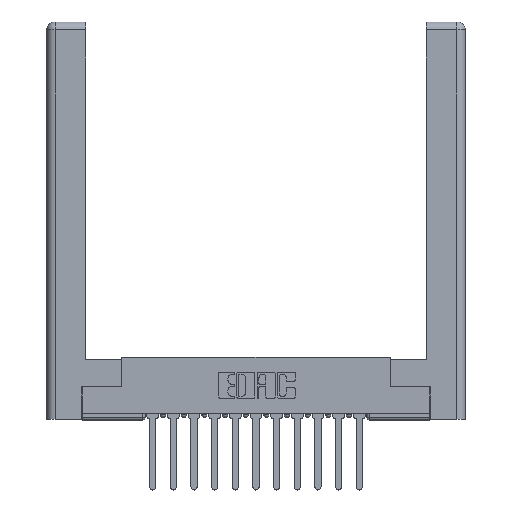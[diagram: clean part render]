
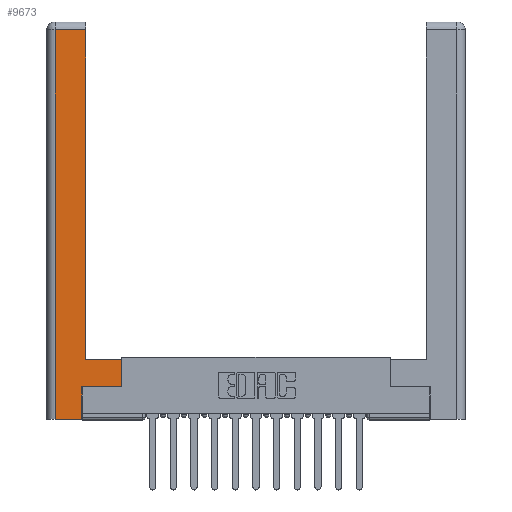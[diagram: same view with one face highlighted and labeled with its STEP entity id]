
A CAD part, top view. The second image highlights one B-rep face of the part: STEP entity #9673.
In plain terms, the highlighted planar face has unit normal (0, 0, 1).
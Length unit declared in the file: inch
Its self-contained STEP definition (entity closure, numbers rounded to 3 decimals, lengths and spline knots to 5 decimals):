
#400 = CARTESIAN_POINT ( 'NONE',  ( 0.565, 0.245, 0. ) ) ;
#1052 = DIRECTION ( 'NONE',  ( 0., 1., 0. ) ) ;
#1970 = CARTESIAN_POINT ( 'NONE',  ( 0.265, 0., 0. ) ) ;
#2134 = DIRECTION ( 'NONE',  ( 0., 1., 0. ) ) ;
#2205 = ORIENTED_EDGE ( 'NONE', *, *, #2290, .T. ) ;
#2249 = EDGE_CURVE ( 'NONE', #7767, #11733, #14508, .T. ) ;
#2290 = EDGE_CURVE ( 'NONE', #13692, #11675, #14270, .T. ) ;
#2493 = CARTESIAN_POINT ( 'NONE',  ( 0.565, 0.45, 0. ) ) ;
#2501 = CARTESIAN_POINT ( 'NONE',  ( 0.0615, 0., 0. ) ) ;
#3147 = EDGE_CURVE ( 'NONE', #8965, #13692, #14709, .T. ) ;
#3248 = FACE_OUTER_BOUND ( 'NONE', #9506, .T. ) ;
#3335 = DIRECTION ( 'NONE',  ( 1., 0., 0. ) ) ;
#3465 = CARTESIAN_POINT ( 'NONE',  ( 0.265, 0.245, 0. ) ) ;
#3655 = EDGE_CURVE ( 'NONE', #11675, #15448, #3921, .T. ) ;
#3697 = CARTESIAN_POINT ( 'NONE',  ( 0.295, 0.45, 0. ) ) ;
#3921 = LINE ( 'NONE', #12734, #9464 ) ;
#3983 = ORIENTED_EDGE ( 'NONE', *, *, #14773, .T. ) ;
#4382 = DIRECTION ( 'NONE',  ( 0., 0., -1. ) ) ;
#4872 = ORIENTED_EDGE ( 'NONE', *, *, #3147, .T. ) ;
#6028 = DIRECTION ( 'NONE',  ( -1., 0., 0. ) ) ;
#6265 = LINE ( 'NONE', #400, #9743 ) ;
#6908 = ORIENTED_EDGE ( 'NONE', *, *, #2249, .T. ) ;
#7004 = VECTOR ( 'NONE', #6028, 39.37008 ) ;
#7348 = VECTOR ( 'NONE', #3335, 39.37008 ) ;
#7767 = VERTEX_POINT ( 'NONE', #2501 ) ;
#8149 = DIRECTION ( 'NONE',  ( -1., 0., 0. ) ) ;
#8499 = VECTOR ( 'NONE', #9912, 39.37008 ) ;
#8590 = CARTESIAN_POINT ( 'NONE',  ( 0.295, 0.45, 0. ) ) ;
#8814 = CARTESIAN_POINT ( 'NONE',  ( 0.0615, 2.94, 0. ) ) ;
#8965 = VERTEX_POINT ( 'NONE', #2493 ) ;
#8978 = ORIENTED_EDGE ( 'NONE', *, *, #3655, .T. ) ;
#9109 = EDGE_CURVE ( 'NONE', #13355, #11329, #6265, .T. ) ;
#9464 = VECTOR ( 'NONE', #14921, 39.37008 ) ;
#9482 = CARTESIAN_POINT ( 'NONE',  ( 0.565, 0.245, 0. ) ) ;
#9506 = EDGE_LOOP ( 'NONE', ( #2205, #8978, #9710, #6908, #3983, #10526, #13446, #4872 ) ) ;
#9673 = ADVANCED_FACE ( 'NONE', ( #3248 ), #14338, .F. ) ;
#9710 = ORIENTED_EDGE ( 'NONE', *, *, #11186, .T. ) ;
#9743 = VECTOR ( 'NONE', #13891, 39.37008 ) ;
#9912 = DIRECTION ( 'NONE',  ( 0., -1., 0. ) ) ;
#10526 = ORIENTED_EDGE ( 'NONE', *, *, #9109, .T. ) ;
#10554 = CARTESIAN_POINT ( 'NONE',  ( 0., 0., 0. ) ) ;
#11186 = EDGE_CURVE ( 'NONE', #15448, #7767, #11418, .T. ) ;
#11329 = VERTEX_POINT ( 'NONE', #9482 ) ;
#11418 = LINE ( 'NONE', #14080, #8499 ) ;
#11473 = CARTESIAN_POINT ( 'NONE',  ( 0.295, 2.94, 0. ) ) ;
#11481 = LINE ( 'NONE', #13904, #15697 ) ;
#11675 = VERTEX_POINT ( 'NONE', #11473 ) ;
#11733 = VERTEX_POINT ( 'NONE', #14303 ) ;
#11758 = CARTESIAN_POINT ( 'NONE',  ( 0.295, 3., 0. ) ) ;
#12154 = EDGE_CURVE ( 'NONE', #11329, #8965, #11481, .T. ) ;
#12574 = AXIS2_PLACEMENT_3D ( 'NONE', #10554, #4382, #8149 ) ;
#12734 = CARTESIAN_POINT ( 'NONE',  ( 0.0615, 2.94, 0. ) ) ;
#13355 = VERTEX_POINT ( 'NONE', #15041 ) ;
#13446 = ORIENTED_EDGE ( 'NONE', *, *, #12154, .T. ) ;
#13692 = VERTEX_POINT ( 'NONE', #3697 ) ;
#13891 = DIRECTION ( 'NONE',  ( 1., 0., 0. ) ) ;
#13904 = CARTESIAN_POINT ( 'NONE',  ( 0.565, 0.45, 0. ) ) ;
#13988 = DIRECTION ( 'NONE',  ( 0., 1., 0. ) ) ;
#14015 = VECTOR ( 'NONE', #2134, 39.37008 ) ;
#14080 = CARTESIAN_POINT ( 'NONE',  ( 0.0615, 0., 0. ) ) ;
#14270 = LINE ( 'NONE', #11758, #14015 ) ;
#14303 = CARTESIAN_POINT ( 'NONE',  ( 0.265, 0., 0. ) ) ;
#14338 = PLANE ( 'NONE',  #12574 ) ;
#14499 = VECTOR ( 'NONE', #1052, 39.37008 ) ;
#14508 = LINE ( 'NONE', #1970, #7348 ) ;
#14709 = LINE ( 'NONE', #8590, #7004 ) ;
#14773 = EDGE_CURVE ( 'NONE', #11733, #13355, #15741, .T. ) ;
#14921 = DIRECTION ( 'NONE',  ( -1., 0., 0. ) ) ;
#15041 = CARTESIAN_POINT ( 'NONE',  ( 0.265, 0.245, 0. ) ) ;
#15448 = VERTEX_POINT ( 'NONE', #8814 ) ;
#15697 = VECTOR ( 'NONE', #13988, 39.37008 ) ;
#15741 = LINE ( 'NONE', #3465, #14499 ) ;
